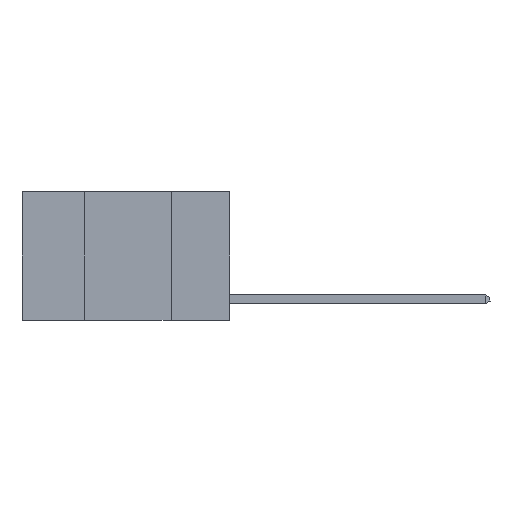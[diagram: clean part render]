
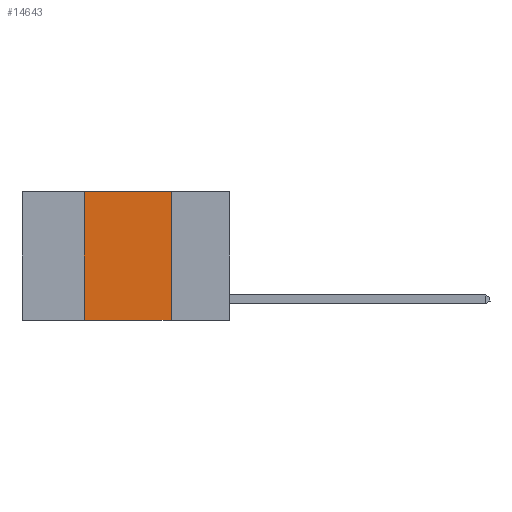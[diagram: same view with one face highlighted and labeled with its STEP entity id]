
A CAD part, left-side view. The second image highlights one B-rep face of the part: STEP entity #14643.
In plain terms, the highlighted planar face has unit normal (-1, 0, 0).
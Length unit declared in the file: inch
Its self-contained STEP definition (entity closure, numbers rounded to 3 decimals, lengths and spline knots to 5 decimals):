
#2097 = VERTEX_POINT ( 'NONE', #13886 ) ;
#4269 = CARTESIAN_POINT ( 'NONE',  ( 0., 0.42, -0.37 ) ) ;
#4974 = CARTESIAN_POINT ( 'NONE',  ( 0., 0.42, 0. ) ) ;
#4986 = VERTEX_POINT ( 'NONE', #21811 ) ;
#5059 = EDGE_CURVE ( 'NONE', #2097, #4986, #14895, .T. ) ;
#5393 = EDGE_CURVE ( 'NONE', #6834, #4986, #17549, .T. ) ;
#5561 = ORIENTED_EDGE ( 'NONE', *, *, #5393, .T. ) ;
#6109 = ORIENTED_EDGE ( 'NONE', *, *, #5059, .F. ) ;
#6282 = EDGE_LOOP ( 'NONE', ( #6109, #21352, #8900, #5561 ) ) ;
#6389 = EDGE_CURVE ( 'NONE', #6834, #20454, #12923, .T. ) ;
#6542 = CARTESIAN_POINT ( 'NONE',  ( 0., 0.17, 0. ) ) ;
#6834 = VERTEX_POINT ( 'NONE', #4269 ) ;
#6907 = CARTESIAN_POINT ( 'NONE',  ( 0., 0.6, 0. ) ) ;
#8900 = ORIENTED_EDGE ( 'NONE', *, *, #6389, .F. ) ;
#9652 = FACE_OUTER_BOUND ( 'NONE', #6282, .T. ) ;
#10344 = VECTOR ( 'NONE', #22041, 39.37008 ) ;
#10364 = DIRECTION ( 'NONE',  ( 0., 0., -1. ) ) ;
#11553 = EDGE_CURVE ( 'NONE', #20454, #2097, #19753, .T. ) ;
#12795 = DIRECTION ( 'NONE',  ( 0., -1., 0. ) ) ;
#12923 = LINE ( 'NONE', #4974, #14022 ) ;
#12966 = VECTOR ( 'NONE', #12795, 39.37008 ) ;
#13886 = CARTESIAN_POINT ( 'NONE',  ( 0., 0.17, 0. ) ) ;
#14022 = VECTOR ( 'NONE', #22145, 39.37008 ) ;
#14643 = ADVANCED_FACE ( 'NONE', ( #9652 ), #17178, .F. ) ;
#14895 = LINE ( 'NONE', #6542, #10344 ) ;
#15571 = CARTESIAN_POINT ( 'NONE',  ( 0., 0.6, 0. ) ) ;
#15717 = VECTOR ( 'NONE', #17285, 39.37008 ) ;
#16196 = CARTESIAN_POINT ( 'NONE',  ( 0., 0.6, -0.37 ) ) ;
#17178 = PLANE ( 'NONE',  #17378 ) ;
#17285 = DIRECTION ( 'NONE',  ( 0., -1., 0. ) ) ;
#17378 = AXIS2_PLACEMENT_3D ( 'NONE', #6907, #20643, #10364 ) ;
#17549 = LINE ( 'NONE', #16196, #12966 ) ;
#19753 = LINE ( 'NONE', #15571, #15717 ) ;
#20454 = VERTEX_POINT ( 'NONE', #22193 ) ;
#20643 = DIRECTION ( 'NONE',  ( 1., 0., 0. ) ) ;
#21352 = ORIENTED_EDGE ( 'NONE', *, *, #11553, .F. ) ;
#21811 = CARTESIAN_POINT ( 'NONE',  ( 0., 0.17, -0.37 ) ) ;
#22041 = DIRECTION ( 'NONE',  ( 0., 0., -1. ) ) ;
#22145 = DIRECTION ( 'NONE',  ( 0., 0., 1. ) ) ;
#22193 = CARTESIAN_POINT ( 'NONE',  ( 0., 0.42, 0. ) ) ;
